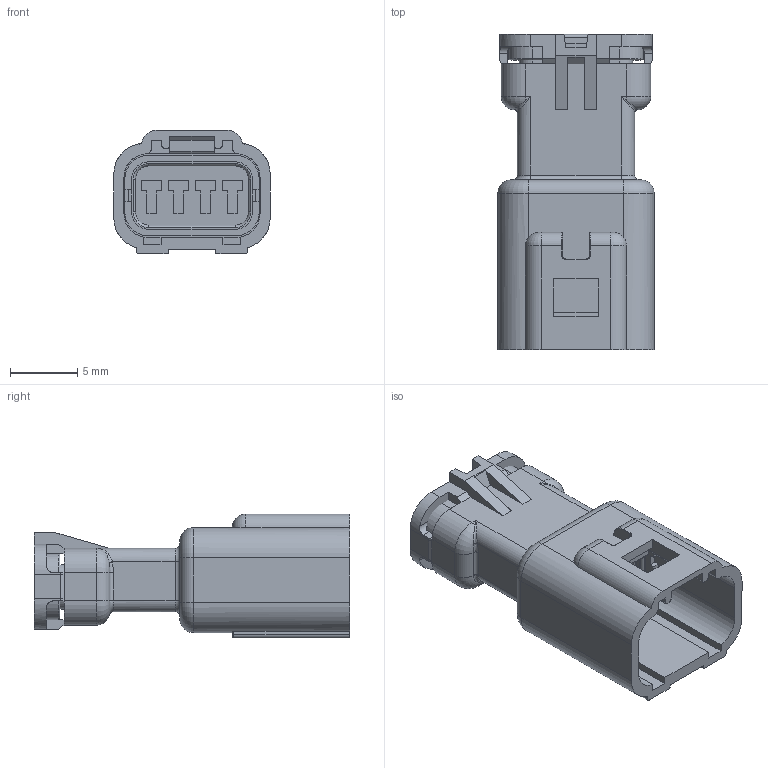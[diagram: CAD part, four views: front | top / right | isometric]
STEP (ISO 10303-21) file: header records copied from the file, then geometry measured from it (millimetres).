
FILE_DESCRIPTION (( 'STEP AP203' ), '1' );
FILE_NAME ('566-004-000-710.STEP', '2021-10-08T13:40:27', ( '' ), ( '' ), 'SwSTEP 2.0', 'SolidWorks 2020', '' );
FILE_SCHEMA (( 'CONFIG_CONTROL_DESIGN' ));
Length unit declared in the file: millimetre
Products named in the file (1): 566-004-000-710
Bounding box: 11.6 x 23.4 x 9.2 mm (x, y, z)
Volume: 932.4 mm3; surface area: 2186.3 mm2
Topology: 2 solids, 3 shells, 763 faces, 2056 edges, 1296 vertices
Faces by surface type: plane 416, cylinder 237, torus 80, bspline 12, sphere 10, cone 8
Entity records: 24143 total; most frequent: CARTESIAN_POINT 4742, ORIENTED_EDGE 4088, DIRECTION 4016, EDGE_CURVE 2044, LINE 1388, VECTOR 1388, AXIS2_PLACEMENT_3D 1314, VERTEX_POINT 1296
